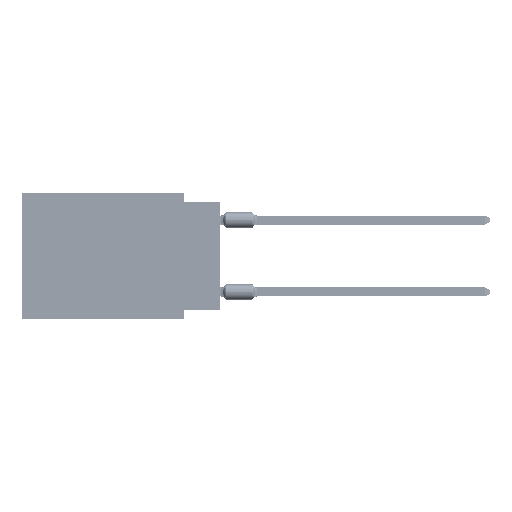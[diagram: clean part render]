
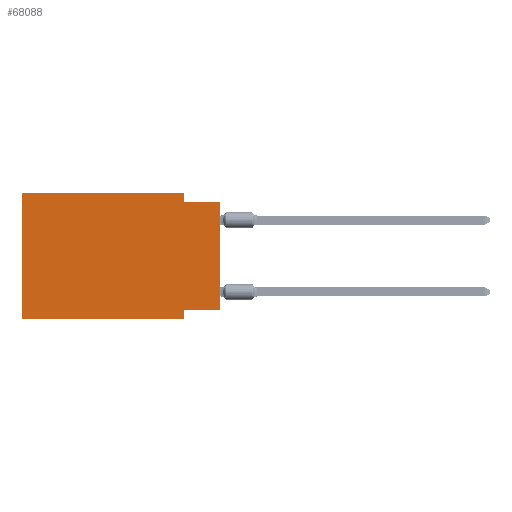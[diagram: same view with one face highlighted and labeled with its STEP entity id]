
A CAD part, left-side view. The second image highlights one B-rep face of the part: STEP entity #68088.
In plain terms, the highlighted planar face has unit normal (-1, 0, 0).
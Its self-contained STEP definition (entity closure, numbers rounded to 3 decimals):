
#1289 = CARTESIAN_POINT ( 'NONE',  ( 0., 0., 0. ) ) ;
#2053 = LINE ( 'NONE', #13408, #68400 ) ;
#3933 = ORIENTED_EDGE ( 'NONE', *, *, #53461, .F. ) ;
#5780 = DIRECTION ( 'NONE',  ( 1., 0., 0. ) ) ;
#6270 = EDGE_CURVE ( 'NONE', #104629, #16564, #28060, .T. ) ;
#10042 = EDGE_LOOP ( 'NONE', ( #57769, #38172, #76552, #3933, #90303, #14280, #92040, #101232 ) ) ;
#12269 = DIRECTION ( 'NONE',  ( 0., -1., 0. ) ) ;
#13408 = CARTESIAN_POINT ( 'NONE',  ( 0., 13.97, -8.89 ) ) ;
#14280 = ORIENTED_EDGE ( 'NONE', *, *, #78023, .T. ) ;
#15984 = CARTESIAN_POINT ( 'NONE',  ( 0., 0., -0.635 ) ) ;
#16564 = VERTEX_POINT ( 'NONE', #93076 ) ;
#20487 = VERTEX_POINT ( 'NONE', #23186 ) ;
#21119 = LINE ( 'NONE', #105092, #81300 ) ;
#22985 = VERTEX_POINT ( 'NONE', #93378 ) ;
#23142 = VECTOR ( 'NONE', #26286, 1000. ) ;
#23186 = CARTESIAN_POINT ( 'NONE',  ( 0., 2.54, -0.635 ) ) ;
#23802 = PLANE ( 'NONE',  #67044 ) ;
#26286 = DIRECTION ( 'NONE',  ( 0., 0., -1. ) ) ;
#27282 = LINE ( 'NONE', #117329, #95348 ) ;
#28060 = LINE ( 'NONE', #91102, #23142 ) ;
#29835 = VERTEX_POINT ( 'NONE', #86613 ) ;
#31984 = CARTESIAN_POINT ( 'NONE',  ( 0., 0., -8.255 ) ) ;
#32172 = CARTESIAN_POINT ( 'NONE',  ( 0., 13.97, 0. ) ) ;
#32811 = CARTESIAN_POINT ( 'NONE',  ( 0., 0., -0.635 ) ) ;
#36324 = LINE ( 'NONE', #109556, #51865 ) ;
#38172 = ORIENTED_EDGE ( 'NONE', *, *, #75329, .F. ) ;
#45857 = VERTEX_POINT ( 'NONE', #15984 ) ;
#49398 = LINE ( 'NONE', #31984, #58536 ) ;
#51865 = VECTOR ( 'NONE', #56133, 1000. ) ;
#52507 = EDGE_CURVE ( 'NONE', #112711, #104629, #49398, .T. ) ;
#53461 = EDGE_CURVE ( 'NONE', #29835, #67863, #27282, .T. ) ;
#56133 = DIRECTION ( 'NONE',  ( 0., 0., -1. ) ) ;
#57704 = DIRECTION ( 'NONE',  ( 0., 0., 1. ) ) ;
#57769 = ORIENTED_EDGE ( 'NONE', *, *, #117662, .T. ) ;
#58536 = VECTOR ( 'NONE', #86005, 1000. ) ;
#60817 = EDGE_CURVE ( 'NONE', #67863, #20487, #36324, .T. ) ;
#61656 = VECTOR ( 'NONE', #93087, 1000. ) ;
#67044 = AXIS2_PLACEMENT_3D ( 'NONE', #32172, #5780, #97003 ) ;
#67863 = VERTEX_POINT ( 'NONE', #72592 ) ;
#68088 = ADVANCED_FACE ( 'NONE', ( #107768 ), #23802, .F. ) ;
#68400 = VECTOR ( 'NONE', #12269, 1000. ) ;
#71864 = VECTOR ( 'NONE', #78428, 1000. ) ;
#72592 = CARTESIAN_POINT ( 'NONE',  ( 0., 2.54, 0. ) ) ;
#75329 = EDGE_CURVE ( 'NONE', #20487, #45857, #77263, .T. ) ;
#76552 = ORIENTED_EDGE ( 'NONE', *, *, #60817, .F. ) ;
#77263 = LINE ( 'NONE', #32811, #71864 ) ;
#78023 = EDGE_CURVE ( 'NONE', #22985, #16564, #2053, .T. ) ;
#78428 = DIRECTION ( 'NONE',  ( 0., -1., 0. ) ) ;
#80127 = DIRECTION ( 'NONE',  ( 0., -1., 0. ) ) ;
#81300 = VECTOR ( 'NONE', #57704, 1000. ) ;
#83484 = LINE ( 'NONE', #1289, #61656 ) ;
#86005 = DIRECTION ( 'NONE',  ( 0., 1., 0. ) ) ;
#86613 = CARTESIAN_POINT ( 'NONE',  ( 0., 13.97, 0. ) ) ;
#90303 = ORIENTED_EDGE ( 'NONE', *, *, #99307, .F. ) ;
#91102 = CARTESIAN_POINT ( 'NONE',  ( 0., 2.54, -8.89 ) ) ;
#92040 = ORIENTED_EDGE ( 'NONE', *, *, #6270, .F. ) ;
#93076 = CARTESIAN_POINT ( 'NONE',  ( 0., 2.54, -8.89 ) ) ;
#93087 = DIRECTION ( 'NONE',  ( 0., 0., 1. ) ) ;
#93378 = CARTESIAN_POINT ( 'NONE',  ( 0., 13.97, -8.89 ) ) ;
#95348 = VECTOR ( 'NONE', #80127, 1000. ) ;
#97003 = DIRECTION ( 'NONE',  ( 0., 0., -1. ) ) ;
#98926 = CARTESIAN_POINT ( 'NONE',  ( 0., 0., -8.255 ) ) ;
#99307 = EDGE_CURVE ( 'NONE', #22985, #29835, #21119, .T. ) ;
#101232 = ORIENTED_EDGE ( 'NONE', *, *, #52507, .F. ) ;
#104629 = VERTEX_POINT ( 'NONE', #112296 ) ;
#105092 = CARTESIAN_POINT ( 'NONE',  ( 0., 13.97, 0. ) ) ;
#107768 = FACE_OUTER_BOUND ( 'NONE', #10042, .T. ) ;
#109556 = CARTESIAN_POINT ( 'NONE',  ( 0., 2.54, 0. ) ) ;
#112296 = CARTESIAN_POINT ( 'NONE',  ( 0., 2.54, -8.255 ) ) ;
#112711 = VERTEX_POINT ( 'NONE', #98926 ) ;
#117329 = CARTESIAN_POINT ( 'NONE',  ( 0., 13.97, 0. ) ) ;
#117662 = EDGE_CURVE ( 'NONE', #112711, #45857, #83484, .T. ) ;
